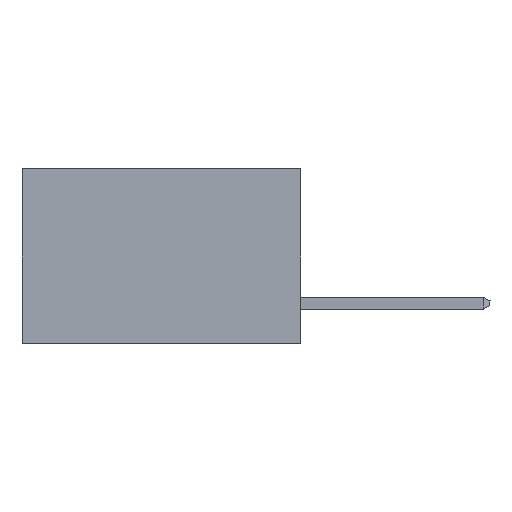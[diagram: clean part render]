
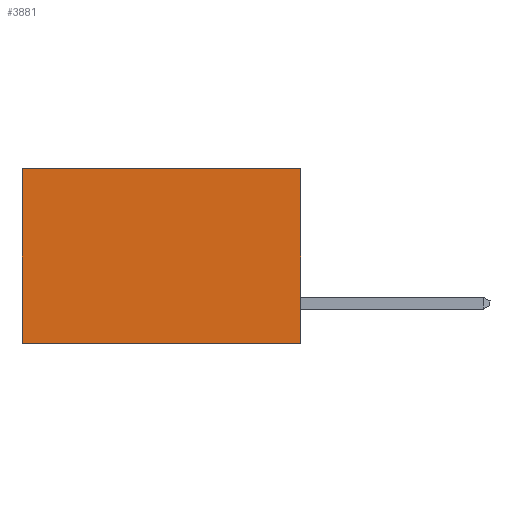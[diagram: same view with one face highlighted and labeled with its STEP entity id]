
A CAD part, left-side view. The second image highlights one B-rep face of the part: STEP entity #3881.
In plain terms, the highlighted planar face has unit normal (-1, 0, 0).
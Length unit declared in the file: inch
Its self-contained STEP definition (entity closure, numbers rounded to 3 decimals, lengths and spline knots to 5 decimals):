
#600 = VERTEX_POINT ( 'NONE', #12012 ) ;
#1021 = DIRECTION ( 'NONE',  ( 0., 0., -1. ) ) ;
#1078 = CARTESIAN_POINT ( 'NONE',  ( 0.277, 0.59, 0. ) ) ;
#1244 = ORIENTED_EDGE ( 'NONE', *, *, #18013, .T. ) ;
#2128 = DIRECTION ( 'NONE',  ( 0., 0., -1. ) ) ;
#2153 = DIRECTION ( 'NONE',  ( 1., 0., 0. ) ) ;
#2385 = CARTESIAN_POINT ( 'NONE',  ( 0.277, 0., -0.37 ) ) ;
#2709 = VECTOR ( 'NONE', #11734, 39.37008 ) ;
#2721 = AXIS2_PLACEMENT_3D ( 'NONE', #2385, #2153, #2128 ) ;
#3024 = CARTESIAN_POINT ( 'NONE',  ( 0.277, 0.59, -0.37 ) ) ;
#3342 = VECTOR ( 'NONE', #9437, 39.37008 ) ;
#3433 = PLANE ( 'NONE',  #2721 ) ;
#3541 = LINE ( 'NONE', #10300, #15858 ) ;
#3881 = ADVANCED_FACE ( 'NONE', ( #7244 ), #3433, .F. ) ;
#5457 = VERTEX_POINT ( 'NONE', #8248 ) ;
#7244 = FACE_OUTER_BOUND ( 'NONE', #8146, .T. ) ;
#7528 = EDGE_CURVE ( 'NONE', #600, #9956, #7978, .T. ) ;
#7978 = LINE ( 'NONE', #9484, #3342 ) ;
#8146 = EDGE_LOOP ( 'NONE', ( #9722, #12924, #15239, #1244 ) ) ;
#8208 = VERTEX_POINT ( 'NONE', #1078 ) ;
#8248 = CARTESIAN_POINT ( 'NONE',  ( 0.277, 0., 0. ) ) ;
#8549 = EDGE_CURVE ( 'NONE', #8208, #9956, #3541, .T. ) ;
#9437 = DIRECTION ( 'NONE',  ( 0., 1., 0. ) ) ;
#9484 = CARTESIAN_POINT ( 'NONE',  ( 0.277, 0., -0.37 ) ) ;
#9722 = ORIENTED_EDGE ( 'NONE', *, *, #8549, .T. ) ;
#9956 = VERTEX_POINT ( 'NONE', #3024 ) ;
#10300 = CARTESIAN_POINT ( 'NONE',  ( 0.277, 0.59, -0.37 ) ) ;
#11211 = VECTOR ( 'NONE', #11319, 39.37008 ) ;
#11319 = DIRECTION ( 'NONE',  ( 0., 1., 0. ) ) ;
#11734 = DIRECTION ( 'NONE',  ( 0., 0., -1. ) ) ;
#12012 = CARTESIAN_POINT ( 'NONE',  ( 0.277, 0., -0.37 ) ) ;
#12924 = ORIENTED_EDGE ( 'NONE', *, *, #7528, .F. ) ;
#15029 = LINE ( 'NONE', #19403, #2709 ) ;
#15239 = ORIENTED_EDGE ( 'NONE', *, *, #19421, .F. ) ;
#15772 = LINE ( 'NONE', #18986, #11211 ) ;
#15858 = VECTOR ( 'NONE', #1021, 39.37008 ) ;
#18013 = EDGE_CURVE ( 'NONE', #5457, #8208, #15772, .T. ) ;
#18986 = CARTESIAN_POINT ( 'NONE',  ( 0.277, 0., 0. ) ) ;
#19403 = CARTESIAN_POINT ( 'NONE',  ( 0.277, 0., -0.37 ) ) ;
#19421 = EDGE_CURVE ( 'NONE', #5457, #600, #15029, .T. ) ;
